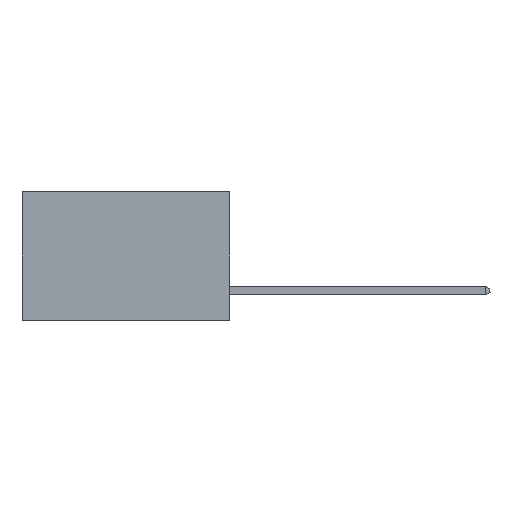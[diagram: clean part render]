
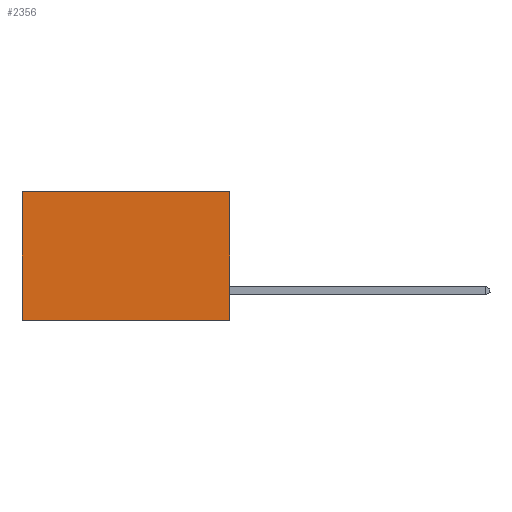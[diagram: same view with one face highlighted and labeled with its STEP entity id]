
A CAD part, left-side view. The second image highlights one B-rep face of the part: STEP entity #2356.
In plain terms, the highlighted planar face has unit normal (-1, 0, 0).
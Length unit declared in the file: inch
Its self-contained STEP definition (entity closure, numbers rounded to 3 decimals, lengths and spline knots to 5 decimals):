
#22 = CARTESIAN_POINT ( 'NONE',  ( 0.298, 0.6, 0. ) ) ;
#475 = EDGE_CURVE ( 'NONE', #16304, #18233, #7635, .T. ) ;
#583 = VECTOR ( 'NONE', #5310, 39.37008 ) ;
#934 = CARTESIAN_POINT ( 'NONE',  ( 0.298, 0., 0. ) ) ;
#1796 = CARTESIAN_POINT ( 'NONE',  ( 0.298, 0., 0. ) ) ;
#2329 = LINE ( 'NONE', #7568, #11972 ) ;
#2356 = ADVANCED_FACE ( 'NONE', ( #11068 ), #13991, .F. ) ;
#3465 = VERTEX_POINT ( 'NONE', #20156 ) ;
#3604 = EDGE_CURVE ( 'NONE', #16304, #3465, #5927, .T. ) ;
#4779 = DIRECTION ( 'NONE',  ( 1., 0., 0. ) ) ;
#5310 = DIRECTION ( 'NONE',  ( 0., 1., 0. ) ) ;
#5314 = ORIENTED_EDGE ( 'NONE', *, *, #28851, .F. ) ;
#5927 = LINE ( 'NONE', #934, #583 ) ;
#6285 = ORIENTED_EDGE ( 'NONE', *, *, #475, .F. ) ;
#6411 = EDGE_CURVE ( 'NONE', #3465, #20527, #9714, .T. ) ;
#7003 = ORIENTED_EDGE ( 'NONE', *, *, #3604, .T. ) ;
#7568 = CARTESIAN_POINT ( 'NONE',  ( 0.298, 0., -0.37 ) ) ;
#7635 = LINE ( 'NONE', #1796, #28482 ) ;
#9714 = LINE ( 'NONE', #22, #11880 ) ;
#10034 = DIRECTION ( 'NONE',  ( 0., 0., -1. ) ) ;
#10544 = ORIENTED_EDGE ( 'NONE', *, *, #6411, .T. ) ;
#11068 = FACE_OUTER_BOUND ( 'NONE', #23232, .T. ) ;
#11880 = VECTOR ( 'NONE', #27406, 39.37008 ) ;
#11972 = VECTOR ( 'NONE', #23715, 39.37008 ) ;
#13096 = CARTESIAN_POINT ( 'NONE',  ( 0.298, 0.6, -0.37 ) ) ;
#13991 = PLANE ( 'NONE',  #23163 ) ;
#16186 = DIRECTION ( 'NONE',  ( 0., 0., -1. ) ) ;
#16304 = VERTEX_POINT ( 'NONE', #19624 ) ;
#18233 = VERTEX_POINT ( 'NONE', #26733 ) ;
#19624 = CARTESIAN_POINT ( 'NONE',  ( 0.298, 0., 0. ) ) ;
#20156 = CARTESIAN_POINT ( 'NONE',  ( 0.298, 0.6, 0. ) ) ;
#20527 = VERTEX_POINT ( 'NONE', #13096 ) ;
#23163 = AXIS2_PLACEMENT_3D ( 'NONE', #23226, #4779, #16186 ) ;
#23226 = CARTESIAN_POINT ( 'NONE',  ( 0.298, 0., 0. ) ) ;
#23232 = EDGE_LOOP ( 'NONE', ( #10544, #5314, #6285, #7003 ) ) ;
#23715 = DIRECTION ( 'NONE',  ( 0., 1., 0. ) ) ;
#26733 = CARTESIAN_POINT ( 'NONE',  ( 0.298, 0., -0.37 ) ) ;
#27406 = DIRECTION ( 'NONE',  ( 0., 0., -1. ) ) ;
#28482 = VECTOR ( 'NONE', #10034, 39.37008 ) ;
#28851 = EDGE_CURVE ( 'NONE', #18233, #20527, #2329, .T. ) ;
